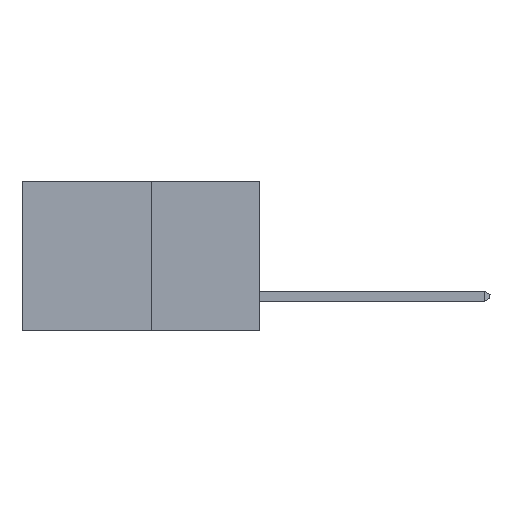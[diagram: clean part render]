
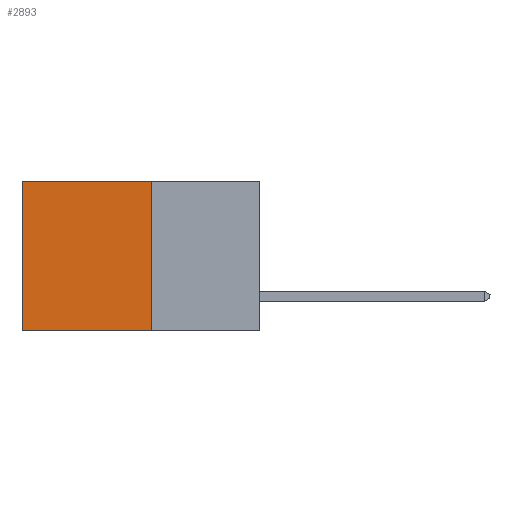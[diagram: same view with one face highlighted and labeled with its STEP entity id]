
A CAD part, left-side view. The second image highlights one B-rep face of the part: STEP entity #2893.
In plain terms, the highlighted planar face has unit normal (-1, 0, 0).
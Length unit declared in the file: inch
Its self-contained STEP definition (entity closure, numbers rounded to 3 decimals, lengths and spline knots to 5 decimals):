
#19 = DIRECTION ( 'NONE',  ( 0., 0., -1. ) ) ;
#389 = VECTOR ( 'NONE', #8062, 39.37008 ) ;
#666 = LINE ( 'NONE', #7607, #389 ) ;
#1112 = VERTEX_POINT ( 'NONE', #10531 ) ;
#1441 = LINE ( 'NONE', #2000, #3606 ) ;
#1580 = DIRECTION ( 'NONE',  ( 0., 0., -1. ) ) ;
#1610 = DIRECTION ( 'NONE',  ( 0., 1., 0. ) ) ;
#1685 = CARTESIAN_POINT ( 'NONE',  ( 0.277, 0.27, -0.37 ) ) ;
#1734 = DIRECTION ( 'NONE',  ( 1., 0., 0. ) ) ;
#1963 = DIRECTION ( 'NONE',  ( 0., 0., -1. ) ) ;
#1967 = CARTESIAN_POINT ( 'NONE',  ( 0.277, 0.27, -0.37 ) ) ;
#2000 = CARTESIAN_POINT ( 'NONE',  ( 0.277, 0.59, -0.37 ) ) ;
#2004 = EDGE_CURVE ( 'NONE', #6571, #9201, #666, .T. ) ;
#2085 = PLANE ( 'NONE',  #5541 ) ;
#2893 = ADVANCED_FACE ( 'NONE', ( #8565 ), #2085, .F. ) ;
#3361 = VECTOR ( 'NONE', #1610, 39.37008 ) ;
#3606 = VECTOR ( 'NONE', #1963, 39.37008 ) ;
#5211 = EDGE_LOOP ( 'NONE', ( #6919, #6678, #6680, #8607 ) ) ;
#5541 = AXIS2_PLACEMENT_3D ( 'NONE', #1967, #1734, #1580 ) ;
#5800 = EDGE_CURVE ( 'NONE', #6571, #1112, #6831, .T. ) ;
#6571 = VERTEX_POINT ( 'NONE', #10038 ) ;
#6576 = VECTOR ( 'NONE', #19, 39.37008 ) ;
#6678 = ORIENTED_EDGE ( 'NONE', *, *, #8290, .F. ) ;
#6680 = ORIENTED_EDGE ( 'NONE', *, *, #5800, .F. ) ;
#6831 = LINE ( 'NONE', #6994, #6576 ) ;
#6919 = ORIENTED_EDGE ( 'NONE', *, *, #7665, .T. ) ;
#6994 = CARTESIAN_POINT ( 'NONE',  ( 0.277, 0.27, -0.37 ) ) ;
#7607 = CARTESIAN_POINT ( 'NONE',  ( 0.277, 0.27, 0. ) ) ;
#7665 = EDGE_CURVE ( 'NONE', #9201, #7682, #1441, .T. ) ;
#7682 = VERTEX_POINT ( 'NONE', #8648 ) ;
#8062 = DIRECTION ( 'NONE',  ( 0., 1., 0. ) ) ;
#8063 = CARTESIAN_POINT ( 'NONE',  ( 0.277, 0.59, 0. ) ) ;
#8290 = EDGE_CURVE ( 'NONE', #1112, #7682, #9738, .T. ) ;
#8565 = FACE_OUTER_BOUND ( 'NONE', #5211, .T. ) ;
#8607 = ORIENTED_EDGE ( 'NONE', *, *, #2004, .T. ) ;
#8648 = CARTESIAN_POINT ( 'NONE',  ( 0.277, 0.59, -0.37 ) ) ;
#9201 = VERTEX_POINT ( 'NONE', #8063 ) ;
#9738 = LINE ( 'NONE', #1685, #3361 ) ;
#10038 = CARTESIAN_POINT ( 'NONE',  ( 0.277, 0.27, 0. ) ) ;
#10531 = CARTESIAN_POINT ( 'NONE',  ( 0.277, 0.27, -0.37 ) ) ;
